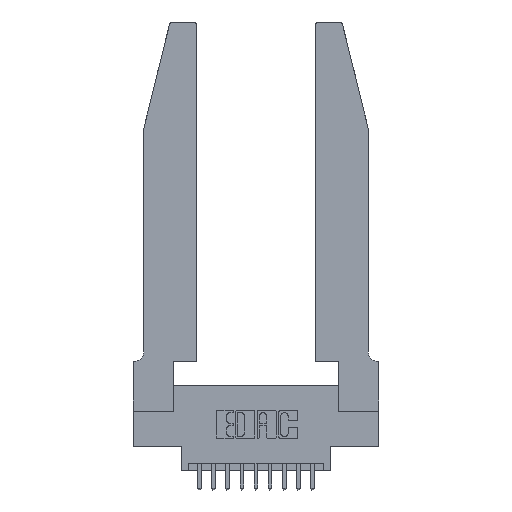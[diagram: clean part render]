
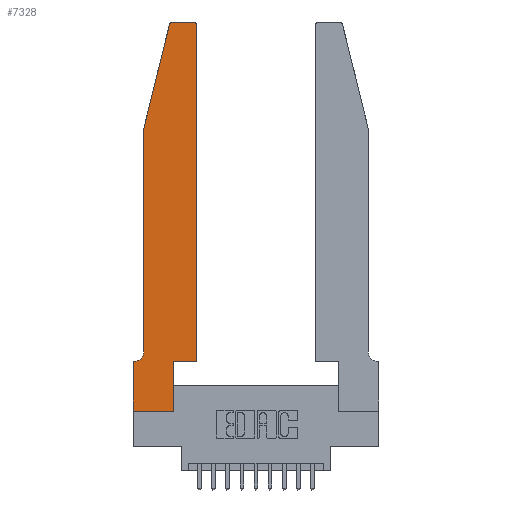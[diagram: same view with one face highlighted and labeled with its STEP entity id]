
A CAD part, top view. The second image highlights one B-rep face of the part: STEP entity #7328.
In plain terms, the highlighted planar face has unit normal (0, 0, 1).
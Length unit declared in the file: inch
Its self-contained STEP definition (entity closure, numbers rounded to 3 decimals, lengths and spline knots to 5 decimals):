
#71 = CIRCLE ( 'NONE', #8881, 0.03 ) ;
#447 = VECTOR ( 'NONE', #15150, 39.37008 ) ;
#458 = DIRECTION ( 'NONE',  ( 0., 0., 1. ) ) ;
#1341 = EDGE_CURVE ( 'NONE', #10430, #7098, #10442, .T. ) ;
#1750 = LINE ( 'NONE', #2076, #12202 ) ;
#1818 = DIRECTION ( 'NONE',  ( -0.239, -0.971, 0. ) ) ;
#1831 = DIRECTION ( 'NONE',  ( 1., 0., 0. ) ) ;
#2076 = CARTESIAN_POINT ( 'NONE',  ( 0., 0., 0.37 ) ) ;
#2388 = VECTOR ( 'NONE', #11301, 39.37008 ) ;
#2589 = CARTESIAN_POINT ( 'NONE',  ( 0.2865, 0., 0.37 ) ) ;
#2730 = CARTESIAN_POINT ( 'NONE',  ( 0.4205, 2.72, 0.37 ) ) ;
#2952 = CARTESIAN_POINT ( 'NONE',  ( 0.0755, 0.35, 0.37 ) ) ;
#3011 = CARTESIAN_POINT ( 'NONE',  ( 0.284, 2.72, 0.37 ) ) ;
#3070 = ORIENTED_EDGE ( 'NONE', *, *, #10904, .T. ) ;
#3096 = PLANE ( 'NONE',  #10948 ) ;
#3247 = VERTEX_POINT ( 'NONE', #7460 ) ;
#3263 = CARTESIAN_POINT ( 'NONE',  ( 0.0055, 0.35, 0.37 ) ) ;
#3356 = EDGE_CURVE ( 'NONE', #3776, #10430, #1750, .T. ) ;
#3632 = LINE ( 'NONE', #2952, #9841 ) ;
#3768 = CARTESIAN_POINT ( 'NONE',  ( 0., 0., 0.37 ) ) ;
#3776 = VERTEX_POINT ( 'NONE', #13797 ) ;
#3966 = VERTEX_POINT ( 'NONE', #3263 ) ;
#4392 = CARTESIAN_POINT ( 'NONE',  ( 0.0755, 0.42, 0.37 ) ) ;
#4399 = EDGE_CURVE ( 'NONE', #3247, #5357, #7640, .T. ) ;
#4456 = DIRECTION ( 'NONE',  ( 0., -1., 0. ) ) ;
#4514 = LINE ( 'NONE', #4671, #5314 ) ;
#4671 = CARTESIAN_POINT ( 'NONE',  ( 0.2865, 0.35, 0.37 ) ) ;
#4738 = VERTEX_POINT ( 'NONE', #10140 ) ;
#4903 = VERTEX_POINT ( 'NONE', #11993 ) ;
#5314 = VECTOR ( 'NONE', #15683, 39.37008 ) ;
#5357 = VERTEX_POINT ( 'NONE', #4392 ) ;
#5475 = CARTESIAN_POINT ( 'NONE',  ( 0.0055, 0.42, 0.37 ) ) ;
#5674 = ORIENTED_EDGE ( 'NONE', *, *, #16304, .T. ) ;
#6387 = CARTESIAN_POINT ( 'NONE',  ( 0.2605, 2.75, 0.37 ) ) ;
#6582 = ORIENTED_EDGE ( 'NONE', *, *, #7585, .T. ) ;
#6621 = CARTESIAN_POINT ( 'NONE',  ( 0.4205, 2.75, 0.37 ) ) ;
#6778 = ORIENTED_EDGE ( 'NONE', *, *, #14365, .T. ) ;
#6948 = DIRECTION ( 'NONE',  ( -1., 0., 0. ) ) ;
#6996 = AXIS2_PLACEMENT_3D ( 'NONE', #5475, #15572, #7992 ) ;
#7057 = LINE ( 'NONE', #12363, #8630 ) ;
#7098 = VERTEX_POINT ( 'NONE', #2589 ) ;
#7150 = VECTOR ( 'NONE', #16290, 39.37008 ) ;
#7328 = ADVANCED_FACE ( 'NONE', ( #10409 ), #3096, .T. ) ;
#7366 = CARTESIAN_POINT ( 'NONE',  ( 0.4505, 0.35, 0.37 ) ) ;
#7460 = CARTESIAN_POINT ( 'NONE',  ( 0.0755, 2., 0.37 ) ) ;
#7585 = EDGE_CURVE ( 'NONE', #3966, #3776, #3632, .T. ) ;
#7640 = LINE ( 'NONE', #15800, #16025 ) ;
#7709 = EDGE_CURVE ( 'NONE', #4903, #4738, #8900, .T. ) ;
#7992 = DIRECTION ( 'NONE',  ( -1., 0., 0. ) ) ;
#8017 = CARTESIAN_POINT ( 'NONE',  ( 0.25487, 2.72718, 0.37 ) ) ;
#8133 = CARTESIAN_POINT ( 'NONE',  ( 0., 0.35, 0.37 ) ) ;
#8157 = ORIENTED_EDGE ( 'NONE', *, *, #1341, .T. ) ;
#8409 = EDGE_CURVE ( 'NONE', #10283, #3247, #9267, .T. ) ;
#8491 = DIRECTION ( 'NONE',  ( 0., 1., 0. ) ) ;
#8630 = VECTOR ( 'NONE', #8491, 39.37008 ) ;
#8660 = LINE ( 'NONE', #6387, #2388 ) ;
#8875 = ORIENTED_EDGE ( 'NONE', *, *, #8993, .T. ) ;
#8881 = AXIS2_PLACEMENT_3D ( 'NONE', #2730, #15561, #10424 ) ;
#8900 = LINE ( 'NONE', #7366, #7150 ) ;
#8993 = EDGE_CURVE ( 'NONE', #5357, #3966, #9239, .T. ) ;
#9239 = CIRCLE ( 'NONE', #6996, 0.07 ) ;
#9267 = LINE ( 'NONE', #9519, #13485 ) ;
#9483 = ORIENTED_EDGE ( 'NONE', *, *, #8409, .T. ) ;
#9519 = CARTESIAN_POINT ( 'NONE',  ( 0.0755, 2., 0.37 ) ) ;
#9546 = CARTESIAN_POINT ( 'NONE',  ( 0.284, 2.75, 0.37 ) ) ;
#9841 = VECTOR ( 'NONE', #6948, 39.37008 ) ;
#10140 = CARTESIAN_POINT ( 'NONE',  ( 0.4505, 0.35, 0.37 ) ) ;
#10261 = CARTESIAN_POINT ( 'NONE',  ( 0., 0., 0.37 ) ) ;
#10283 = VERTEX_POINT ( 'NONE', #8017 ) ;
#10409 = FACE_OUTER_BOUND ( 'NONE', #11899, .T. ) ;
#10424 = DIRECTION ( 'NONE',  ( 1., 0., 0. ) ) ;
#10430 = VERTEX_POINT ( 'NONE', #10261 ) ;
#10442 = LINE ( 'NONE', #3768, #447 ) ;
#10728 = DIRECTION ( 'NONE',  ( 1., 0., 0. ) ) ;
#10904 = EDGE_CURVE ( 'NONE', #7098, #4903, #4514, .T. ) ;
#10948 = AXIS2_PLACEMENT_3D ( 'NONE', #8133, #15819, #10728 ) ;
#10975 = EDGE_CURVE ( 'NONE', #4738, #16228, #7057, .T. ) ;
#11301 = DIRECTION ( 'NONE',  ( -1., 0., 0. ) ) ;
#11430 = AXIS2_PLACEMENT_3D ( 'NONE', #3011, #458, #1831 ) ;
#11899 = EDGE_LOOP ( 'NONE', ( #14405, #5674, #9483, #14214, #8875, #6582, #14456, #8157, #3070, #14438, #12659, #6778 ) ) ;
#11993 = CARTESIAN_POINT ( 'NONE',  ( 0.2865, 0.35, 0.37 ) ) ;
#12202 = VECTOR ( 'NONE', #4456, 39.37008 ) ;
#12363 = CARTESIAN_POINT ( 'NONE',  ( 0.4505, 0.35, 0.37 ) ) ;
#12659 = ORIENTED_EDGE ( 'NONE', *, *, #10975, .T. ) ;
#13485 = VECTOR ( 'NONE', #1818, 39.37008 ) ;
#13797 = CARTESIAN_POINT ( 'NONE',  ( 0., 0.35, 0.37 ) ) ;
#13804 = CIRCLE ( 'NONE', #11430, 0.03 ) ;
#14214 = ORIENTED_EDGE ( 'NONE', *, *, #4399, .T. ) ;
#14353 = VERTEX_POINT ( 'NONE', #6621 ) ;
#14365 = EDGE_CURVE ( 'NONE', #16228, #14353, #71, .T. ) ;
#14405 = ORIENTED_EDGE ( 'NONE', *, *, #14916, .T. ) ;
#14438 = ORIENTED_EDGE ( 'NONE', *, *, #7709, .T. ) ;
#14456 = ORIENTED_EDGE ( 'NONE', *, *, #3356, .T. ) ;
#14723 = DIRECTION ( 'NONE',  ( 0., -1., 0. ) ) ;
#14916 = EDGE_CURVE ( 'NONE', #14353, #15704, #8660, .T. ) ;
#15150 = DIRECTION ( 'NONE',  ( 1., 0., 0. ) ) ;
#15515 = CARTESIAN_POINT ( 'NONE',  ( 0.4505, 2.72, 0.37 ) ) ;
#15561 = DIRECTION ( 'NONE',  ( 0., 0., 1. ) ) ;
#15572 = DIRECTION ( 'NONE',  ( 0., 0., -1. ) ) ;
#15683 = DIRECTION ( 'NONE',  ( 0., 1., 0. ) ) ;
#15704 = VERTEX_POINT ( 'NONE', #9546 ) ;
#15800 = CARTESIAN_POINT ( 'NONE',  ( 0.0755, 2., 0.37 ) ) ;
#15819 = DIRECTION ( 'NONE',  ( 0., 0., 1. ) ) ;
#16025 = VECTOR ( 'NONE', #14723, 39.37008 ) ;
#16228 = VERTEX_POINT ( 'NONE', #15515 ) ;
#16290 = DIRECTION ( 'NONE',  ( 1., 0., 0. ) ) ;
#16304 = EDGE_CURVE ( 'NONE', #15704, #10283, #13804, .T. ) ;
